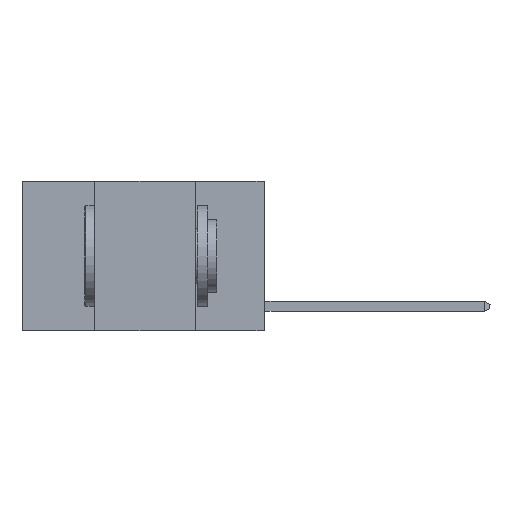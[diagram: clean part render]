
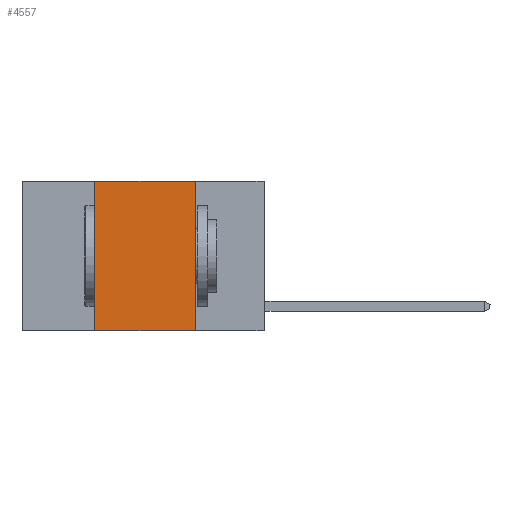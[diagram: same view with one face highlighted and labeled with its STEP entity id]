
A CAD part, left-side view. The second image highlights one B-rep face of the part: STEP entity #4557.
In plain terms, the highlighted planar face has unit normal (-1, 0, 0).
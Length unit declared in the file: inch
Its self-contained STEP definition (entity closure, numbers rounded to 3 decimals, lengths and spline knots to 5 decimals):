
#74 = CARTESIAN_POINT ( 'NONE',  ( 0., 0.17, -0.37 ) ) ;
#212 = CARTESIAN_POINT ( 'NONE',  ( 0., 0.42, 0. ) ) ;
#492 = VERTEX_POINT ( 'NONE', #74 ) ;
#1627 = VERTEX_POINT ( 'NONE', #8811 ) ;
#1736 = CARTESIAN_POINT ( 'NONE',  ( 0., 0.17, 0. ) ) ;
#2575 = VECTOR ( 'NONE', #12749, 39.37008 ) ;
#2642 = FACE_OUTER_BOUND ( 'NONE', #5198, .T. ) ;
#3700 = ORIENTED_EDGE ( 'NONE', *, *, #6171, .T. ) ;
#4399 = DIRECTION ( 'NONE',  ( 0., -1., 0. ) ) ;
#4556 = LINE ( 'NONE', #5433, #7003 ) ;
#4557 = ADVANCED_FACE ( 'NONE', ( #2642 ), #11828, .F. ) ;
#4592 = AXIS2_PLACEMENT_3D ( 'NONE', #11992, #11655, #11594 ) ;
#5033 = LINE ( 'NONE', #5659, #2575 ) ;
#5198 = EDGE_LOOP ( 'NONE', ( #6160, #8897, #11600, #3700 ) ) ;
#5433 = CARTESIAN_POINT ( 'NONE',  ( 0., 0.6, 0. ) ) ;
#5659 = CARTESIAN_POINT ( 'NONE',  ( 0., 0.42, 0. ) ) ;
#5742 = VECTOR ( 'NONE', #9085, 39.37008 ) ;
#5876 = LINE ( 'NONE', #9604, #11321 ) ;
#5879 = VERTEX_POINT ( 'NONE', #1736 ) ;
#6160 = ORIENTED_EDGE ( 'NONE', *, *, #8932, .F. ) ;
#6171 = EDGE_CURVE ( 'NONE', #1627, #492, #5876, .T. ) ;
#7003 = VECTOR ( 'NONE', #4399, 39.37008 ) ;
#7545 = DIRECTION ( 'NONE',  ( 0., -1., 0. ) ) ;
#7548 = EDGE_CURVE ( 'NONE', #1627, #9855, #5033, .T. ) ;
#8811 = CARTESIAN_POINT ( 'NONE',  ( 0., 0.42, -0.37 ) ) ;
#8897 = ORIENTED_EDGE ( 'NONE', *, *, #10551, .F. ) ;
#8932 = EDGE_CURVE ( 'NONE', #5879, #492, #11192, .T. ) ;
#9085 = DIRECTION ( 'NONE',  ( 0., 0., -1. ) ) ;
#9604 = CARTESIAN_POINT ( 'NONE',  ( 0., 0.6, -0.37 ) ) ;
#9855 = VERTEX_POINT ( 'NONE', #212 ) ;
#10084 = CARTESIAN_POINT ( 'NONE',  ( 0., 0.17, 0. ) ) ;
#10551 = EDGE_CURVE ( 'NONE', #9855, #5879, #4556, .T. ) ;
#11192 = LINE ( 'NONE', #10084, #5742 ) ;
#11321 = VECTOR ( 'NONE', #7545, 39.37008 ) ;
#11594 = DIRECTION ( 'NONE',  ( 0., 0., -1. ) ) ;
#11600 = ORIENTED_EDGE ( 'NONE', *, *, #7548, .F. ) ;
#11655 = DIRECTION ( 'NONE',  ( 1., 0., 0. ) ) ;
#11828 = PLANE ( 'NONE',  #4592 ) ;
#11992 = CARTESIAN_POINT ( 'NONE',  ( 0., 0.6, 0. ) ) ;
#12749 = DIRECTION ( 'NONE',  ( 0., 0., 1. ) ) ;
